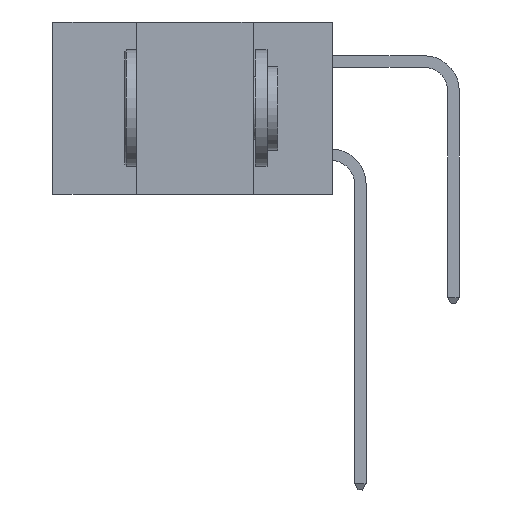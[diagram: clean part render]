
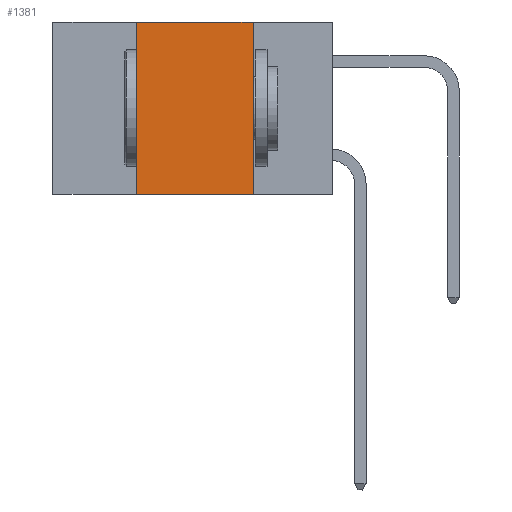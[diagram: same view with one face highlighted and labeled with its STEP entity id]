
A CAD part, left-side view. The second image highlights one B-rep face of the part: STEP entity #1381.
In plain terms, the highlighted planar face has unit normal (-1, 0, 0).
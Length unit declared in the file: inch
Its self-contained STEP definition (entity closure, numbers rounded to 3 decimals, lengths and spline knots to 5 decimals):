
#625 = DIRECTION ( 'NONE',  ( 0., -1., 0. ) ) ;
#921 = DIRECTION ( 'NONE',  ( 1., 0., 0. ) ) ;
#1223 = FACE_OUTER_BOUND ( 'NONE', #10242, .T. ) ;
#1381 = ADVANCED_FACE ( 'NONE', ( #1223 ), #12524, .F. ) ;
#1462 = ORIENTED_EDGE ( 'NONE', *, *, #7689, .T. ) ;
#1535 = VECTOR ( 'NONE', #8006, 39.37008 ) ;
#1685 = VERTEX_POINT ( 'NONE', #16143 ) ;
#2081 = CARTESIAN_POINT ( 'NONE',  ( 0., 0.6, -0.37 ) ) ;
#2366 = EDGE_CURVE ( 'NONE', #21481, #6879, #25475, .T. ) ;
#2590 = CARTESIAN_POINT ( 'NONE',  ( 0., 0.42, -0.37 ) ) ;
#2647 = ORIENTED_EDGE ( 'NONE', *, *, #22677, .F. ) ;
#2944 = ORIENTED_EDGE ( 'NONE', *, *, #2366, .F. ) ;
#4366 = DIRECTION ( 'NONE',  ( 0., 0., -1. ) ) ;
#6879 = VERTEX_POINT ( 'NONE', #23029 ) ;
#7689 = EDGE_CURVE ( 'NONE', #21481, #22969, #18657, .T. ) ;
#8006 = DIRECTION ( 'NONE',  ( 0., 0., 1. ) ) ;
#8441 = CARTESIAN_POINT ( 'NONE',  ( 0., 0.6, 0. ) ) ;
#8822 = VECTOR ( 'NONE', #22993, 39.37008 ) ;
#9041 = CARTESIAN_POINT ( 'NONE',  ( 0., 0.17, -0.37 ) ) ;
#10242 = EDGE_LOOP ( 'NONE', ( #23859, #2647, #2944, #1462 ) ) ;
#12524 = PLANE ( 'NONE',  #14318 ) ;
#13179 = VECTOR ( 'NONE', #625, 39.37008 ) ;
#13428 = EDGE_CURVE ( 'NONE', #1685, #22969, #25908, .T. ) ;
#14318 = AXIS2_PLACEMENT_3D ( 'NONE', #8441, #921, #4366 ) ;
#14800 = VECTOR ( 'NONE', #22874, 39.37008 ) ;
#16143 = CARTESIAN_POINT ( 'NONE',  ( 0., 0.17, 0. ) ) ;
#17473 = CARTESIAN_POINT ( 'NONE',  ( 0., 0.6, 0. ) ) ;
#18657 = LINE ( 'NONE', #2081, #14800 ) ;
#21218 = LINE ( 'NONE', #17473, #13179 ) ;
#21481 = VERTEX_POINT ( 'NONE', #2590 ) ;
#22509 = CARTESIAN_POINT ( 'NONE',  ( 0., 0.42, 0. ) ) ;
#22677 = EDGE_CURVE ( 'NONE', #6879, #1685, #21218, .T. ) ;
#22874 = DIRECTION ( 'NONE',  ( 0., -1., 0. ) ) ;
#22969 = VERTEX_POINT ( 'NONE', #9041 ) ;
#22993 = DIRECTION ( 'NONE',  ( 0., 0., -1. ) ) ;
#23029 = CARTESIAN_POINT ( 'NONE',  ( 0., 0.42, 0. ) ) ;
#23859 = ORIENTED_EDGE ( 'NONE', *, *, #13428, .F. ) ;
#24229 = CARTESIAN_POINT ( 'NONE',  ( 0., 0.17, 0. ) ) ;
#25475 = LINE ( 'NONE', #22509, #1535 ) ;
#25908 = LINE ( 'NONE', #24229, #8822 ) ;
